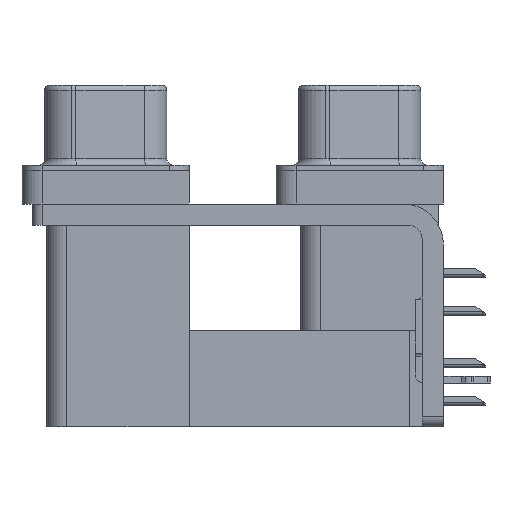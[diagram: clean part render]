
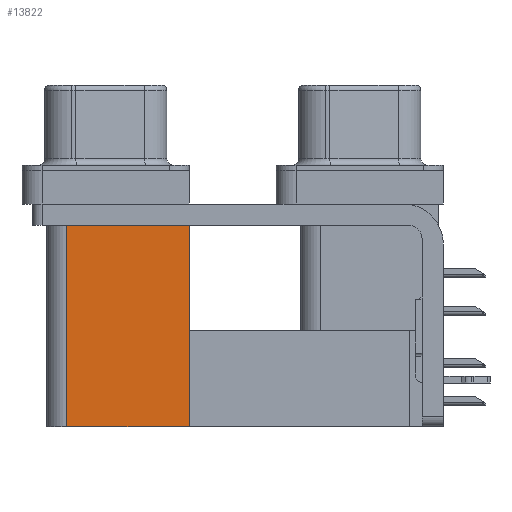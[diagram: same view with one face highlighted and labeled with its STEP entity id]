
A CAD part, left-side view. The second image highlights one B-rep face of the part: STEP entity #13822.
In plain terms, the highlighted planar face has unit normal (-1, 0, 0).
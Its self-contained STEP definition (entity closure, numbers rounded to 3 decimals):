
#537 = DIRECTION ( 'NONE',  ( 1., 0., 0. ) ) ;
#1628 = LINE ( 'NONE', #27204, #26717 ) ;
#3559 = DIRECTION ( 'NONE',  ( 0., 1., 0. ) ) ;
#3707 = DIRECTION ( 'NONE',  ( 0., 0., 1. ) ) ;
#7422 = EDGE_CURVE ( 'NONE', #21311, #32061, #11934, .T. ) ;
#10705 = EDGE_LOOP ( 'NONE', ( #32364, #29160, #31782, #31824 ) ) ;
#10985 = VECTOR ( 'NONE', #29577, 1000. ) ;
#11713 = DIRECTION ( 'NONE',  ( 0., 0., 1. ) ) ;
#11934 = LINE ( 'NONE', #32286, #21289 ) ;
#12163 = VERTEX_POINT ( 'NONE', #30920 ) ;
#12370 = EDGE_CURVE ( 'NONE', #12163, #29792, #1628, .T. ) ;
#13749 = CARTESIAN_POINT ( 'NONE',  ( 3.765, 21.975, -2.5 ) ) ;
#13822 = ADVANCED_FACE ( 'NONE', ( #33146 ), #20355, .F. ) ;
#15500 = CARTESIAN_POINT ( 'NONE',  ( 3.765, 12.775, -19.2 ) ) ;
#20355 = PLANE ( 'NONE',  #23823 ) ;
#21289 = VECTOR ( 'NONE', #3707, 1000. ) ;
#21311 = VERTEX_POINT ( 'NONE', #33191 ) ;
#21663 = LINE ( 'NONE', #31923, #10985 ) ;
#21862 = EDGE_CURVE ( 'NONE', #21311, #12163, #30810, .T. ) ;
#23823 = AXIS2_PLACEMENT_3D ( 'NONE', #30636, #537, #27944 ) ;
#25653 = EDGE_CURVE ( 'NONE', #32061, #29792, #21663, .T. ) ;
#26459 = VECTOR ( 'NONE', #3559, 1000. ) ;
#26640 = CARTESIAN_POINT ( 'NONE',  ( 3.765, 12.775, -2.5 ) ) ;
#26717 = VECTOR ( 'NONE', #11713, 1000. ) ;
#27204 = CARTESIAN_POINT ( 'NONE',  ( 3.765, 21.975, -19.2 ) ) ;
#27944 = DIRECTION ( 'NONE',  ( 0., 0., -1. ) ) ;
#29160 = ORIENTED_EDGE ( 'NONE', *, *, #12370, .F. ) ;
#29577 = DIRECTION ( 'NONE',  ( 0., 1., 0. ) ) ;
#29792 = VERTEX_POINT ( 'NONE', #13749 ) ;
#30636 = CARTESIAN_POINT ( 'NONE',  ( 3.765, 12.775, -19.2 ) ) ;
#30810 = LINE ( 'NONE', #15500, #26459 ) ;
#30920 = CARTESIAN_POINT ( 'NONE',  ( 3.765, 21.975, -19.2 ) ) ;
#31782 = ORIENTED_EDGE ( 'NONE', *, *, #21862, .F. ) ;
#31824 = ORIENTED_EDGE ( 'NONE', *, *, #7422, .T. ) ;
#31923 = CARTESIAN_POINT ( 'NONE',  ( 3.765, 12.775, -2.5 ) ) ;
#32061 = VERTEX_POINT ( 'NONE', #26640 ) ;
#32286 = CARTESIAN_POINT ( 'NONE',  ( 3.765, 12.775, -19.2 ) ) ;
#32364 = ORIENTED_EDGE ( 'NONE', *, *, #25653, .T. ) ;
#33146 = FACE_OUTER_BOUND ( 'NONE', #10705, .T. ) ;
#33191 = CARTESIAN_POINT ( 'NONE',  ( 3.765, 12.775, -19.2 ) ) ;
